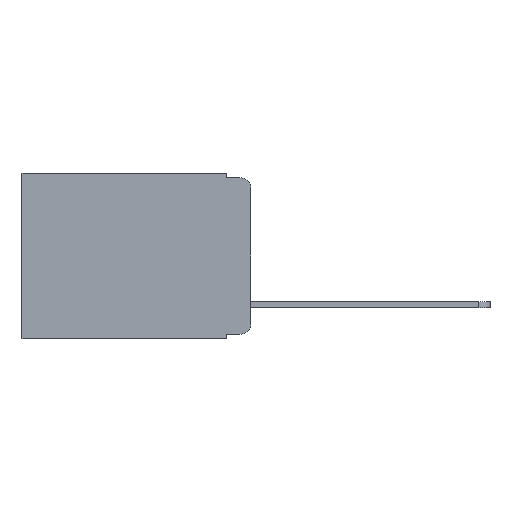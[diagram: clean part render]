
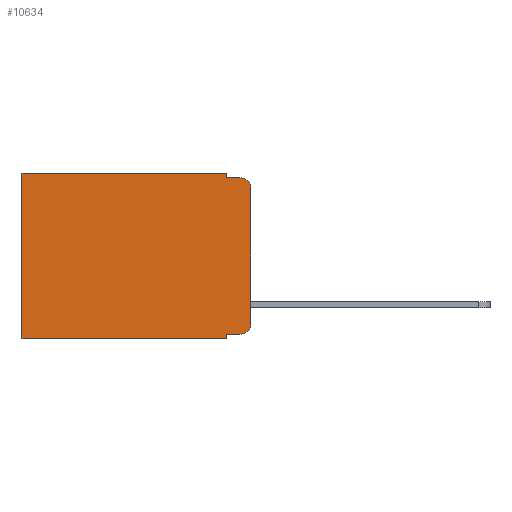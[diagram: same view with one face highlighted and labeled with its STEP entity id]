
A CAD part, left-side view. The second image highlights one B-rep face of the part: STEP entity #10634.
In plain terms, the highlighted planar face has unit normal (-1, 0, 0).
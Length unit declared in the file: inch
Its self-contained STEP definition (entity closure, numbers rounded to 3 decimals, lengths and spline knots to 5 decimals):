
#162 = CARTESIAN_POINT ( 'NONE',  ( 0.298, 0.051, -0.343 ) ) ;
#183 = EDGE_CURVE ( 'NONE', #13558, #8341, #14984, .T. ) ;
#388 = ORIENTED_EDGE ( 'NONE', *, *, #4752, .T. ) ;
#429 = EDGE_CURVE ( 'NONE', #11443, #8341, #15133, .T. ) ;
#582 = CARTESIAN_POINT ( 'NONE',  ( 0.298, 0., -0.343 ) ) ;
#704 = LINE ( 'NONE', #5519, #4019 ) ;
#1161 = CARTESIAN_POINT ( 'NONE',  ( 0.298, 0.051, -0.333 ) ) ;
#1285 = CARTESIAN_POINT ( 'NONE',  ( 0.298, 0., -0.03 ) ) ;
#1489 = VERTEX_POINT ( 'NONE', #5790 ) ;
#1492 = ORIENTED_EDGE ( 'NONE', *, *, #6000, .T. ) ;
#1876 = ORIENTED_EDGE ( 'NONE', *, *, #5682, .F. ) ;
#1898 = CIRCLE ( 'NONE', #9913, 0.02 ) ;
#1933 = DIRECTION ( 'NONE',  ( -1., 0., 0. ) ) ;
#1994 = DIRECTION ( 'NONE',  ( 0., 1., 0. ) ) ;
#2213 = VECTOR ( 'NONE', #11462, 39.37008 ) ;
#2342 = VECTOR ( 'NONE', #12233, 39.37008 ) ;
#2397 = ORIENTED_EDGE ( 'NONE', *, *, #183, .T. ) ;
#2558 = DIRECTION ( 'NONE',  ( 0., 1., 0. ) ) ;
#2681 = CARTESIAN_POINT ( 'NONE',  ( 0.298, 0.051, -0.01 ) ) ;
#2883 = VECTOR ( 'NONE', #6062, 39.37008 ) ;
#3084 = AXIS2_PLACEMENT_3D ( 'NONE', #8155, #5807, #13997 ) ;
#3179 = LINE ( 'NONE', #8920, #6190 ) ;
#3221 = DIRECTION ( 'NONE',  ( 0., -1., 0. ) ) ;
#3395 = ORIENTED_EDGE ( 'NONE', *, *, #13321, .F. ) ;
#3659 = ORIENTED_EDGE ( 'NONE', *, *, #429, .F. ) ;
#3894 = ORIENTED_EDGE ( 'NONE', *, *, #7061, .F. ) ;
#3907 = EDGE_CURVE ( 'NONE', #10396, #1489, #1898, .T. ) ;
#3951 = CARTESIAN_POINT ( 'NONE',  ( 0.298, 0.02, -0.01 ) ) ;
#4019 = VECTOR ( 'NONE', #2558, 39.37008 ) ;
#4158 = VERTEX_POINT ( 'NONE', #11541 ) ;
#4567 = PLANE ( 'NONE',  #3084 ) ;
#4752 = EDGE_CURVE ( 'NONE', #5513, #10396, #3179, .T. ) ;
#4910 = VECTOR ( 'NONE', #1994, 39.37008 ) ;
#5301 = LINE ( 'NONE', #582, #4910 ) ;
#5333 = ORIENTED_EDGE ( 'NONE', *, *, #9114, .F. ) ;
#5446 = CARTESIAN_POINT ( 'NONE',  ( 0.298, 0.473, 0. ) ) ;
#5513 = VERTEX_POINT ( 'NONE', #1161 ) ;
#5519 = CARTESIAN_POINT ( 'NONE',  ( 0.298, 0., 0. ) ) ;
#5568 = EDGE_LOOP ( 'NONE', ( #1876, #2397, #3659, #3894, #1492, #10588, #5333, #3395, #388, #10493 ) ) ;
#5670 = DIRECTION ( 'NONE',  ( 0., 0., -1. ) ) ;
#5682 = EDGE_CURVE ( 'NONE', #13558, #1489, #15073, .T. ) ;
#5729 = VECTOR ( 'NONE', #5670, 39.37008 ) ;
#5740 = LINE ( 'NONE', #6207, #2213 ) ;
#5790 = CARTESIAN_POINT ( 'NONE',  ( 0.298, 0., -0.313 ) ) ;
#5807 = DIRECTION ( 'NONE',  ( 1., 0., 0. ) ) ;
#5935 = LINE ( 'NONE', #13087, #2883 ) ;
#6000 = EDGE_CURVE ( 'NONE', #4158, #11897, #704, .T. ) ;
#6062 = DIRECTION ( 'NONE',  ( 0., 0., -1. ) ) ;
#6190 = VECTOR ( 'NONE', #3221, 39.37008 ) ;
#6207 = CARTESIAN_POINT ( 'NONE',  ( 0.298, 0.051, 0. ) ) ;
#6876 = CARTESIAN_POINT ( 'NONE',  ( 0.298, 0.051, -0.01 ) ) ;
#7061 = EDGE_CURVE ( 'NONE', #4158, #11443, #5740, .T. ) ;
#7369 = EDGE_CURVE ( 'NONE', #11897, #15068, #11977, .T. ) ;
#8155 = CARTESIAN_POINT ( 'NONE',  ( 0.298, 0., 0. ) ) ;
#8341 = VERTEX_POINT ( 'NONE', #3951 ) ;
#8554 = AXIS2_PLACEMENT_3D ( 'NONE', #9372, #1933, #10328 ) ;
#8920 = CARTESIAN_POINT ( 'NONE',  ( 0.298, 0.051, -0.333 ) ) ;
#8954 = VECTOR ( 'NONE', #10881, 39.37008 ) ;
#9114 = EDGE_CURVE ( 'NONE', #10539, #15068, #5301, .T. ) ;
#9304 = CARTESIAN_POINT ( 'NONE',  ( 0.298, 0.02, -0.333 ) ) ;
#9372 = CARTESIAN_POINT ( 'NONE',  ( 0.298, 0.02, -0.03 ) ) ;
#9913 = AXIS2_PLACEMENT_3D ( 'NONE', #13934, #13917, #14002 ) ;
#10328 = DIRECTION ( 'NONE',  ( 0., 0., -1. ) ) ;
#10396 = VERTEX_POINT ( 'NONE', #9304 ) ;
#10493 = ORIENTED_EDGE ( 'NONE', *, *, #3907, .T. ) ;
#10539 = VERTEX_POINT ( 'NONE', #162 ) ;
#10588 = ORIENTED_EDGE ( 'NONE', *, *, #7369, .T. ) ;
#10634 = ADVANCED_FACE ( 'NONE', ( #13892 ), #4567, .F. ) ;
#10881 = DIRECTION ( 'NONE',  ( 0., 0., -1. ) ) ;
#11443 = VERTEX_POINT ( 'NONE', #2681 ) ;
#11462 = DIRECTION ( 'NONE',  ( 0., 0., -1. ) ) ;
#11541 = CARTESIAN_POINT ( 'NONE',  ( 0.298, 0.051, 0. ) ) ;
#11897 = VERTEX_POINT ( 'NONE', #14540 ) ;
#11977 = LINE ( 'NONE', #5446, #5729 ) ;
#12112 = CARTESIAN_POINT ( 'NONE',  ( 0.298, 0., 0. ) ) ;
#12233 = DIRECTION ( 'NONE',  ( 0., -1., 0. ) ) ;
#12650 = CARTESIAN_POINT ( 'NONE',  ( 0.298, 0.473, -0.343 ) ) ;
#13087 = CARTESIAN_POINT ( 'NONE',  ( 0.298, 0.051, 0. ) ) ;
#13321 = EDGE_CURVE ( 'NONE', #5513, #10539, #5935, .T. ) ;
#13558 = VERTEX_POINT ( 'NONE', #1285 ) ;
#13892 = FACE_OUTER_BOUND ( 'NONE', #5568, .T. ) ;
#13917 = DIRECTION ( 'NONE',  ( -1., 0., 0. ) ) ;
#13934 = CARTESIAN_POINT ( 'NONE',  ( 0.298, 0.02, -0.313 ) ) ;
#13997 = DIRECTION ( 'NONE',  ( 0., 0., -1. ) ) ;
#14002 = DIRECTION ( 'NONE',  ( 0., 0., -1. ) ) ;
#14540 = CARTESIAN_POINT ( 'NONE',  ( 0.298, 0.473, 0. ) ) ;
#14984 = CIRCLE ( 'NONE', #8554, 0.02 ) ;
#15068 = VERTEX_POINT ( 'NONE', #12650 ) ;
#15073 = LINE ( 'NONE', #12112, #8954 ) ;
#15133 = LINE ( 'NONE', #6876, #2342 ) ;
